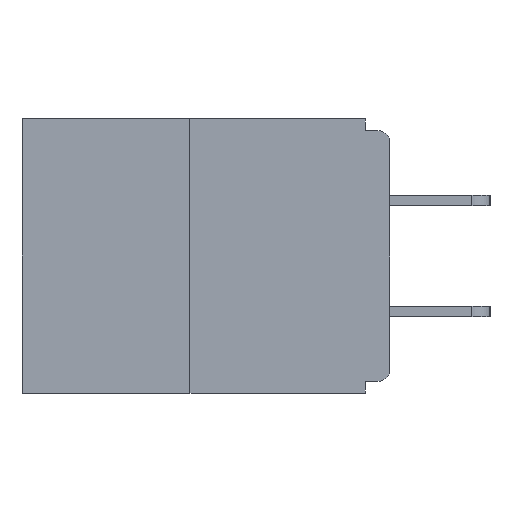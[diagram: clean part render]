
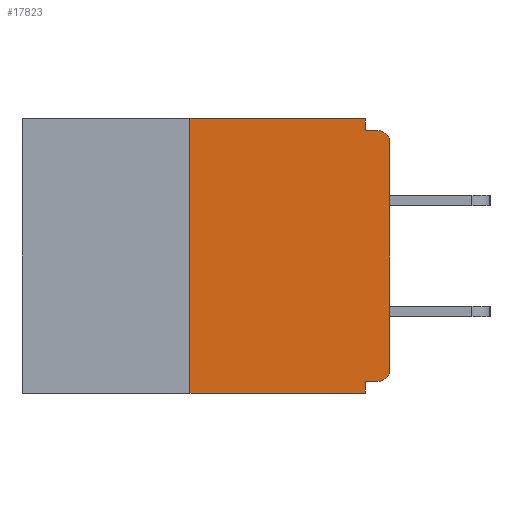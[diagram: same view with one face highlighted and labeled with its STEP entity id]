
A CAD part, left-side view. The second image highlights one B-rep face of the part: STEP entity #17823.
In plain terms, the highlighted planar face has unit normal (-1, 0, 0).
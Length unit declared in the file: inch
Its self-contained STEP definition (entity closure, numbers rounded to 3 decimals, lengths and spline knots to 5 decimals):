
#112 = CARTESIAN_POINT ( 'NONE',  ( 0., 0.25, 0. ) ) ;
#760 = EDGE_CURVE ( 'NONE', #15481, #10327, #4807, .T. ) ;
#808 = AXIS2_PLACEMENT_3D ( 'NONE', #3511, #4845, #5041 ) ;
#1043 = EDGE_CURVE ( 'NONE', #8548, #15481, #15588, .T. ) ;
#1083 = ORIENTED_EDGE ( 'NONE', *, *, #1275, .F. ) ;
#1275 = EDGE_CURVE ( 'NONE', #20664, #7954, #20435, .T. ) ;
#1537 = ORIENTED_EDGE ( 'NONE', *, *, #10980, .F. ) ;
#2403 = ORIENTED_EDGE ( 'NONE', *, *, #760, .F. ) ;
#2821 = AXIS2_PLACEMENT_3D ( 'NONE', #15651, #20620, #20690 ) ;
#2915 = ORIENTED_EDGE ( 'NONE', *, *, #6520, .T. ) ;
#3511 = CARTESIAN_POINT ( 'NONE',  ( 0., 0.46, 0. ) ) ;
#4218 = VECTOR ( 'NONE', #15395, 39.37008 ) ;
#4807 = LINE ( 'NONE', #11208, #17867 ) ;
#4827 = LINE ( 'NONE', #20274, #11077 ) ;
#4845 = DIRECTION ( 'NONE',  ( 1., 0., 0. ) ) ;
#5041 = DIRECTION ( 'NONE',  ( 0., 0., -1. ) ) ;
#5131 = VERTEX_POINT ( 'NONE', #17538 ) ;
#5508 = ORIENTED_EDGE ( 'NONE', *, *, #17456, .F. ) ;
#6520 = EDGE_CURVE ( 'NONE', #19732, #16996, #4827, .T. ) ;
#6790 = EDGE_CURVE ( 'NONE', #5131, #16725, #12094, .T. ) ;
#7954 = VERTEX_POINT ( 'NONE', #18115 ) ;
#8074 = CIRCLE ( 'NONE', #13159, 0.015 ) ;
#8092 = CIRCLE ( 'NONE', #2821, 0.015 ) ;
#8548 = VERTEX_POINT ( 'NONE', #10119 ) ;
#9648 = PLANE ( 'NONE',  #808 ) ;
#9748 = ORIENTED_EDGE ( 'NONE', *, *, #10450, .T. ) ;
#10119 = CARTESIAN_POINT ( 'NONE',  ( 0., 0.015, -0.328 ) ) ;
#10206 = CARTESIAN_POINT ( 'NONE',  ( 0., 0.46, -0.343 ) ) ;
#10327 = VERTEX_POINT ( 'NONE', #19831 ) ;
#10368 = DIRECTION ( 'NONE',  ( 0., 0., 1. ) ) ;
#10440 = ORIENTED_EDGE ( 'NONE', *, *, #19165, .T. ) ;
#10450 = EDGE_CURVE ( 'NONE', #20664, #10327, #13254, .T. ) ;
#10931 = DIRECTION ( 'NONE',  ( 0., 0., -1. ) ) ;
#10954 = CARTESIAN_POINT ( 'NONE',  ( 0., 0.031, 0. ) ) ;
#10980 = EDGE_CURVE ( 'NONE', #20140, #5131, #15994, .T. ) ;
#11077 = VECTOR ( 'NONE', #10368, 39.37008 ) ;
#11105 = CARTESIAN_POINT ( 'NONE',  ( 0., 0., -0.313 ) ) ;
#11208 = CARTESIAN_POINT ( 'NONE',  ( 0., 0.031, -0.343 ) ) ;
#11495 = EDGE_LOOP ( 'NONE', ( #5508, #1083, #9748, #2403, #15504, #10440, #2915, #19718, #20727, #1537 ) ) ;
#11567 = DIRECTION ( 'NONE',  ( 0., 1., 0. ) ) ;
#11783 = CARTESIAN_POINT ( 'NONE',  ( 0., 0., -0.015 ) ) ;
#11923 = DIRECTION ( 'NONE',  ( 0., -1., 0. ) ) ;
#12094 = LINE ( 'NONE', #11783, #16326 ) ;
#13159 = AXIS2_PLACEMENT_3D ( 'NONE', #17503, #14470, #16086 ) ;
#13216 = FACE_OUTER_BOUND ( 'NONE', #11495, .T. ) ;
#13254 = LINE ( 'NONE', #10206, #16757 ) ;
#13323 = DIRECTION ( 'NONE',  ( 0., -1., 0. ) ) ;
#13932 = CARTESIAN_POINT ( 'NONE',  ( 0., 0.015, -0.015 ) ) ;
#14063 = CARTESIAN_POINT ( 'NONE',  ( 0., 0., -0.03 ) ) ;
#14222 = LINE ( 'NONE', #18424, #19825 ) ;
#14470 = DIRECTION ( 'NONE',  ( -1., 0., 0. ) ) ;
#14849 = CARTESIAN_POINT ( 'NONE',  ( 0., 0., -0.328 ) ) ;
#15395 = DIRECTION ( 'NONE',  ( 0., 0., -1. ) ) ;
#15481 = VERTEX_POINT ( 'NONE', #17380 ) ;
#15504 = ORIENTED_EDGE ( 'NONE', *, *, #1043, .F. ) ;
#15588 = LINE ( 'NONE', #14849, #16821 ) ;
#15651 = CARTESIAN_POINT ( 'NONE',  ( 0., 0.015, -0.313 ) ) ;
#15994 = LINE ( 'NONE', #20384, #4218 ) ;
#16081 = VECTOR ( 'NONE', #19484, 39.37008 ) ;
#16086 = DIRECTION ( 'NONE',  ( 0., 0., -1. ) ) ;
#16326 = VECTOR ( 'NONE', #11923, 39.37008 ) ;
#16725 = VERTEX_POINT ( 'NONE', #13932 ) ;
#16757 = VECTOR ( 'NONE', #13323, 39.37008 ) ;
#16821 = VECTOR ( 'NONE', #11567, 39.37008 ) ;
#16996 = VERTEX_POINT ( 'NONE', #14063 ) ;
#17275 = CARTESIAN_POINT ( 'NONE',  ( 0., 0.25, -0.343 ) ) ;
#17380 = CARTESIAN_POINT ( 'NONE',  ( 0., 0.031, -0.328 ) ) ;
#17456 = EDGE_CURVE ( 'NONE', #7954, #20140, #14222, .T. ) ;
#17503 = CARTESIAN_POINT ( 'NONE',  ( 0., 0.015, -0.03 ) ) ;
#17538 = CARTESIAN_POINT ( 'NONE',  ( 0., 0.031, -0.015 ) ) ;
#17823 = ADVANCED_FACE ( 'NONE', ( #13216 ), #9648, .F. ) ;
#17867 = VECTOR ( 'NONE', #10931, 39.37008 ) ;
#18115 = CARTESIAN_POINT ( 'NONE',  ( 0., 0.25, 0. ) ) ;
#18424 = CARTESIAN_POINT ( 'NONE',  ( 0., 0.46, 0. ) ) ;
#18935 = DIRECTION ( 'NONE',  ( 0., -1., 0. ) ) ;
#19165 = EDGE_CURVE ( 'NONE', #8548, #19732, #8092, .T. ) ;
#19484 = DIRECTION ( 'NONE',  ( 0., 0., 1. ) ) ;
#19718 = ORIENTED_EDGE ( 'NONE', *, *, #20198, .T. ) ;
#19732 = VERTEX_POINT ( 'NONE', #11105 ) ;
#19825 = VECTOR ( 'NONE', #18935, 39.37008 ) ;
#19831 = CARTESIAN_POINT ( 'NONE',  ( 0., 0.031, -0.343 ) ) ;
#20140 = VERTEX_POINT ( 'NONE', #10954 ) ;
#20198 = EDGE_CURVE ( 'NONE', #16996, #16725, #8074, .T. ) ;
#20274 = CARTESIAN_POINT ( 'NONE',  ( 0., 0., 0. ) ) ;
#20384 = CARTESIAN_POINT ( 'NONE',  ( 0., 0.031, 0. ) ) ;
#20435 = LINE ( 'NONE', #112, #16081 ) ;
#20620 = DIRECTION ( 'NONE',  ( -1., 0., 0. ) ) ;
#20664 = VERTEX_POINT ( 'NONE', #17275 ) ;
#20690 = DIRECTION ( 'NONE',  ( 0., 0., -1. ) ) ;
#20727 = ORIENTED_EDGE ( 'NONE', *, *, #6790, .F. ) ;
